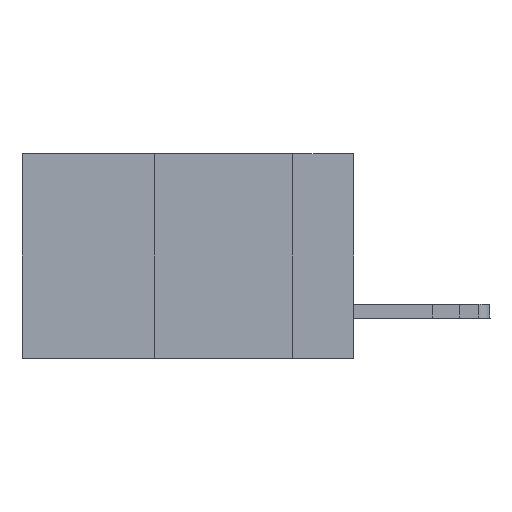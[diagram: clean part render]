
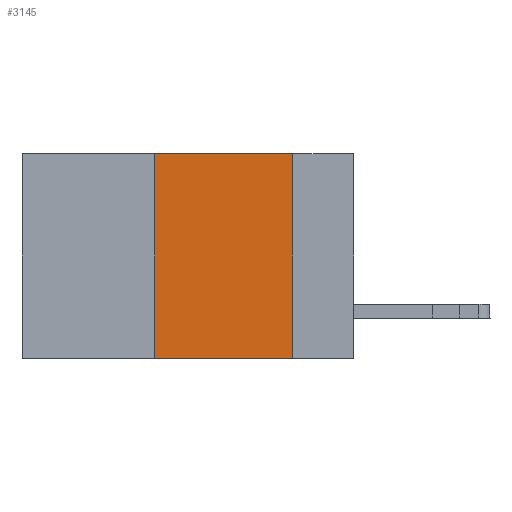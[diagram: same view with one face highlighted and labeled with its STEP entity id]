
A CAD part, left-side view. The second image highlights one B-rep face of the part: STEP entity #3145.
In plain terms, the highlighted planar face has unit normal (-1, 0, 0).
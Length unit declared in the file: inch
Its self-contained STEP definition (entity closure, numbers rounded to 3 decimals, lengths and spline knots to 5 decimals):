
#921 = ORIENTED_EDGE ( 'NONE', *, *, #9498, .T. ) ;
#1255 = PLANE ( 'NONE',  #18736 ) ;
#2091 = EDGE_CURVE ( 'NONE', #27728, #14476, #11584, .T. ) ;
#3145 = ADVANCED_FACE ( 'NONE', ( #3458 ), #1255, .F. ) ;
#3381 = CARTESIAN_POINT ( 'NONE',  ( 0., 0.6, 0. ) ) ;
#3458 = FACE_OUTER_BOUND ( 'NONE', #26420, .T. ) ;
#5495 = ORIENTED_EDGE ( 'NONE', *, *, #10936, .F. ) ;
#6255 = LINE ( 'NONE', #23183, #17661 ) ;
#7750 = CARTESIAN_POINT ( 'NONE',  ( 0., 0.11, 0. ) ) ;
#7924 = DIRECTION ( 'NONE',  ( 0., -1., 0. ) ) ;
#8506 = DIRECTION ( 'NONE',  ( 0., 0., -1. ) ) ;
#8603 = DIRECTION ( 'NONE',  ( 1., 0., 0. ) ) ;
#9089 = EDGE_CURVE ( 'NONE', #24877, #31133, #21425, .T. ) ;
#9498 = EDGE_CURVE ( 'NONE', #27728, #31133, #18371, .T. ) ;
#9930 = DIRECTION ( 'NONE',  ( 0., 0., -1. ) ) ;
#10480 = CARTESIAN_POINT ( 'NONE',  ( 0., 0.11, -0.37 ) ) ;
#10497 = CARTESIAN_POINT ( 'NONE',  ( 0., 0.6, -0.37 ) ) ;
#10936 = EDGE_CURVE ( 'NONE', #14476, #24877, #6255, .T. ) ;
#11584 = LINE ( 'NONE', #23741, #22256 ) ;
#13832 = ORIENTED_EDGE ( 'NONE', *, *, #2091, .F. ) ;
#14166 = VECTOR ( 'NONE', #9930, 39.37008 ) ;
#14476 = VERTEX_POINT ( 'NONE', #29540 ) ;
#17661 = VECTOR ( 'NONE', #25545, 39.37008 ) ;
#18371 = LINE ( 'NONE', #10497, #30632 ) ;
#18736 = AXIS2_PLACEMENT_3D ( 'NONE', #3381, #8603, #8506 ) ;
#21363 = DIRECTION ( 'NONE',  ( 0., 0., 1. ) ) ;
#21425 = LINE ( 'NONE', #24597, #14166 ) ;
#22256 = VECTOR ( 'NONE', #21363, 39.37008 ) ;
#22510 = ORIENTED_EDGE ( 'NONE', *, *, #9089, .F. ) ;
#23183 = CARTESIAN_POINT ( 'NONE',  ( 0., 0.6, 0. ) ) ;
#23741 = CARTESIAN_POINT ( 'NONE',  ( 0., 0.36, 0. ) ) ;
#24597 = CARTESIAN_POINT ( 'NONE',  ( 0., 0.11, 0. ) ) ;
#24877 = VERTEX_POINT ( 'NONE', #7750 ) ;
#25545 = DIRECTION ( 'NONE',  ( 0., -1., 0. ) ) ;
#26420 = EDGE_LOOP ( 'NONE', ( #22510, #5495, #13832, #921 ) ) ;
#27301 = CARTESIAN_POINT ( 'NONE',  ( 0., 0.36, -0.37 ) ) ;
#27728 = VERTEX_POINT ( 'NONE', #27301 ) ;
#29540 = CARTESIAN_POINT ( 'NONE',  ( 0., 0.36, 0. ) ) ;
#30632 = VECTOR ( 'NONE', #7924, 39.37008 ) ;
#31133 = VERTEX_POINT ( 'NONE', #10480 ) ;
